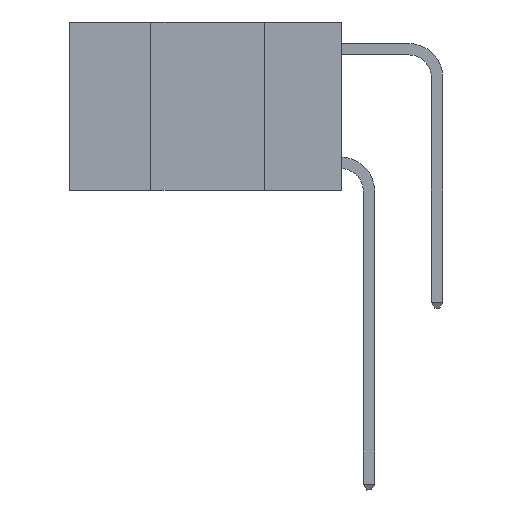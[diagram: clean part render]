
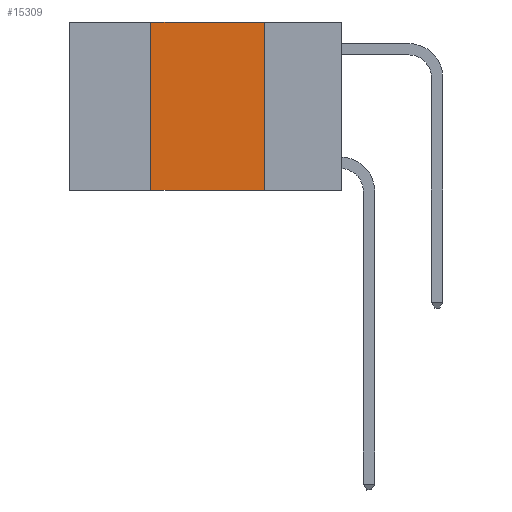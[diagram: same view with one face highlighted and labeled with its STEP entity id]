
A CAD part, left-side view. The second image highlights one B-rep face of the part: STEP entity #15309.
In plain terms, the highlighted planar face has unit normal (-1, 0, 0).
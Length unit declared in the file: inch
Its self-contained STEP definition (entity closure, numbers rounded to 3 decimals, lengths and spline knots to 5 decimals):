
#121 = CARTESIAN_POINT ( 'NONE',  ( 0., 0.42, 0. ) ) ;
#149 = ORIENTED_EDGE ( 'NONE', *, *, #8530, .T. ) ;
#163 = VECTOR ( 'NONE', #15919, 39.37008 ) ;
#1750 = DIRECTION ( 'NONE',  ( 1., 0., 0. ) ) ;
#2467 = AXIS2_PLACEMENT_3D ( 'NONE', #13396, #1750, #6948 ) ;
#3034 = FACE_OUTER_BOUND ( 'NONE', #10745, .T. ) ;
#3346 = LINE ( 'NONE', #13798, #14809 ) ;
#3954 = EDGE_CURVE ( 'NONE', #6011, #7129, #11778, .T. ) ;
#4322 = VECTOR ( 'NONE', #7970, 39.37008 ) ;
#4348 = EDGE_CURVE ( 'NONE', #7129, #15362, #14472, .T. ) ;
#4882 = CARTESIAN_POINT ( 'NONE',  ( 0., 0.17, -0.37 ) ) ;
#4925 = CARTESIAN_POINT ( 'NONE',  ( 0., 0.17, 0. ) ) ;
#5594 = PLANE ( 'NONE',  #2467 ) ;
#6011 = VERTEX_POINT ( 'NONE', #10240 ) ;
#6816 = ORIENTED_EDGE ( 'NONE', *, *, #3954, .F. ) ;
#6818 = CARTESIAN_POINT ( 'NONE',  ( 0., 0.6, 0. ) ) ;
#6948 = DIRECTION ( 'NONE',  ( 0., 0., -1. ) ) ;
#7129 = VERTEX_POINT ( 'NONE', #8129 ) ;
#7430 = ORIENTED_EDGE ( 'NONE', *, *, #4348, .F. ) ;
#7970 = DIRECTION ( 'NONE',  ( 0., 0., 1. ) ) ;
#8030 = CARTESIAN_POINT ( 'NONE',  ( 0., 0.17, 0. ) ) ;
#8129 = CARTESIAN_POINT ( 'NONE',  ( 0., 0.42, 0. ) ) ;
#8530 = EDGE_CURVE ( 'NONE', #6011, #16265, #3346, .T. ) ;
#8870 = EDGE_CURVE ( 'NONE', #15362, #16265, #10815, .T. ) ;
#10240 = CARTESIAN_POINT ( 'NONE',  ( 0., 0.42, -0.37 ) ) ;
#10745 = EDGE_LOOP ( 'NONE', ( #16567, #7430, #6816, #149 ) ) ;
#10815 = LINE ( 'NONE', #8030, #163 ) ;
#11778 = LINE ( 'NONE', #121, #4322 ) ;
#12275 = DIRECTION ( 'NONE',  ( 0., -1., 0. ) ) ;
#13396 = CARTESIAN_POINT ( 'NONE',  ( 0., 0.6, 0. ) ) ;
#13798 = CARTESIAN_POINT ( 'NONE',  ( 0., 0.6, -0.37 ) ) ;
#14472 = LINE ( 'NONE', #6818, #15759 ) ;
#14554 = DIRECTION ( 'NONE',  ( 0., -1., 0. ) ) ;
#14809 = VECTOR ( 'NONE', #12275, 39.37008 ) ;
#15309 = ADVANCED_FACE ( 'NONE', ( #3034 ), #5594, .F. ) ;
#15362 = VERTEX_POINT ( 'NONE', #4925 ) ;
#15759 = VECTOR ( 'NONE', #14554, 39.37008 ) ;
#15919 = DIRECTION ( 'NONE',  ( 0., 0., -1. ) ) ;
#16265 = VERTEX_POINT ( 'NONE', #4882 ) ;
#16567 = ORIENTED_EDGE ( 'NONE', *, *, #8870, .F. ) ;
